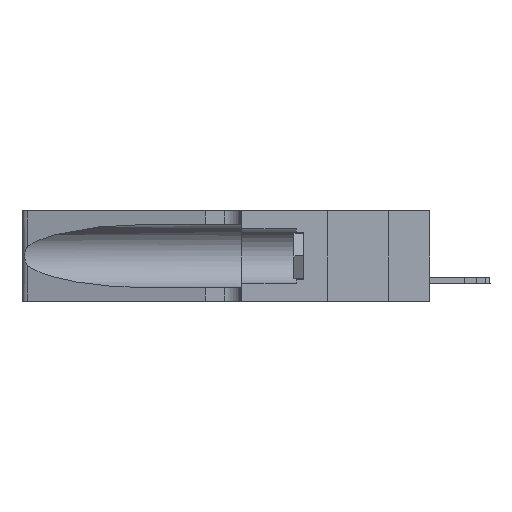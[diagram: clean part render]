
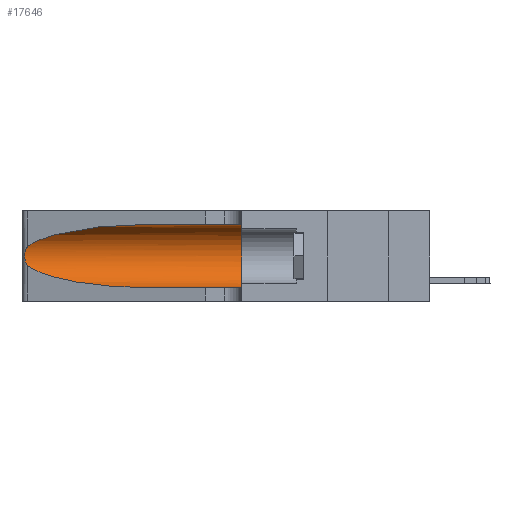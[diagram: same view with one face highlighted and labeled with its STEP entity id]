
A CAD part, left-side view. The second image highlights one B-rep face of the part: STEP entity #17646.
In plain terms, the highlighted cylindrical face has radius 3.308 mm (diameter 6.617 mm), a partial arc.
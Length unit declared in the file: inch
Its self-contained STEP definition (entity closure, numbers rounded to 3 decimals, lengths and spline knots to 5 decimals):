
#485 = ORIENTED_EDGE ( 'NONE', *, *, #11020, .T. ) ;
#548 =( BOUNDED_CURVE ( )  B_SPLINE_CURVE ( 3, ( #13055, #17147, #8443, #1246 ),
 .UNSPECIFIED., .F., .F. ) 
 B_SPLINE_CURVE_WITH_KNOTS ( ( 4, 4 ),
 ( 3.44316, 4.71239 ),
 .UNSPECIFIED. ) 
 CURVE ( )  GEOMETRIC_REPRESENTATION_ITEM ( )  RATIONAL_B_SPLINE_CURVE ( ( 1., 0.87, 0.87, 1. ) ) 
 REPRESENTATION_ITEM ( '' )  );
#1246 = CARTESIAN_POINT ( 'NONE',  ( 0.1305, 0.72297, 0.05475 ) ) ;
#1343 = CARTESIAN_POINT ( 'NONE',  ( 0.26075, 1.23896, 0.19203 ) ) ;
#1542 = CARTESIAN_POINT ( 'NONE',  ( 0.25856, 1.23593, 0.16098 ) ) ;
#1659 = CARTESIAN_POINT ( 'NONE',  ( 0.25487, 1.22718, 0.14631 ) ) ;
#2204 = DIRECTION ( 'NONE',  ( 0., 0., 1. ) ) ;
#2738 = CIRCLE ( 'NONE', #11949, 0.13025 ) ;
#2740 = CARTESIAN_POINT ( 'NONE',  ( 0.18966, 0.96281, 0.31525 ) ) ;
#3016 = VERTEX_POINT ( 'NONE', #12288 ) ;
#4189 = VERTEX_POINT ( 'NONE', #16537 ) ;
#4429 = CARTESIAN_POINT ( 'NONE',  ( 0.25789, 1.23486, 0.15765 ) ) ;
#4461 = EDGE_CURVE ( 'NONE', #3016, #16405, #2738, .T. ) ;
#4575 = CARTESIAN_POINT ( 'NONE',  ( 0.1305, 1.61858, 0.185 ) ) ;
#5717 = CARTESIAN_POINT ( 'NONE',  ( 0.25639, 1.23184, 0.21858 ) ) ;
#6683 = CARTESIAN_POINT ( 'NONE',  ( 0.1305, 0.35, 0.185 ) ) ;
#7173 = DIRECTION ( 'NONE',  ( 0., -1., 0. ) ) ;
#7194 = CARTESIAN_POINT ( 'NONE',  ( 0.25787, 1.23484, 0.2124 ) ) ;
#7376 = CARTESIAN_POINT ( 'NONE',  ( 0.26017, 1.23833, 0.17102 ) ) ;
#7525 = DIRECTION ( 'NONE',  ( 0., 0., -1. ) ) ;
#7537 = VECTOR ( 'NONE', #7173, 39.37008 ) ;
#7862 = LINE ( 'NONE', #10892, #14656 ) ;
#8037 = DIRECTION ( 'NONE',  ( 0., -1., 0. ) ) ;
#8443 = CARTESIAN_POINT ( 'NONE',  ( 0.18966, 0.96281, 0.05475 ) ) ;
#8663 = CARTESIAN_POINT ( 'NONE',  ( 0.25854, 1.2359, 0.20912 ) ) ;
#8679 = CYLINDRICAL_SURFACE ( 'NONE', #16673, 0.13025 ) ;
#9254 = CARTESIAN_POINT ( 'NONE',  ( 0.1305, 0.72297, 0.31525 ) ) ;
#9574 = CARTESIAN_POINT ( 'NONE',  ( 0.1305, 0.35, 0.05475 ) ) ;
#9608 = VERTEX_POINT ( 'NONE', #12617 ) ;
#9744 = EDGE_CURVE ( 'NONE', #11634, #9608, #17561, .T. ) ;
#10396 = ORIENTED_EDGE ( 'NONE', *, *, #11366, .F. ) ;
#10731 = LINE ( 'NONE', #13749, #7537 ) ;
#10815 = VERTEX_POINT ( 'NONE', #1659 ) ;
#10892 = CARTESIAN_POINT ( 'NONE',  ( 0.1305, 1.61858, 0.05475 ) ) ;
#11020 = EDGE_CURVE ( 'NONE', #10815, #4189, #548, .T. ) ;
#11366 = EDGE_CURVE ( 'NONE', #11634, #3016, #10731, .T. ) ;
#11390 = CARTESIAN_POINT ( 'NONE',  ( 0.25487, 1.22718, 0.22369 ) ) ;
#11634 = VERTEX_POINT ( 'NONE', #9254 ) ;
#11896 = EDGE_LOOP ( 'NONE', ( #17261, #17432, #485, #14064, #17115, #10396 ) ) ;
#11949 = AXIS2_PLACEMENT_3D ( 'NONE', #6683, #12455, #2204 ) ;
#12288 = CARTESIAN_POINT ( 'NONE',  ( 0.1305, 0.35, 0.31525 ) ) ;
#12455 = DIRECTION ( 'NONE',  ( 0., 1., 0. ) ) ;
#12617 = CARTESIAN_POINT ( 'NONE',  ( 0.25487, 1.22718, 0.22369 ) ) ;
#12893 = EDGE_CURVE ( 'NONE', #9608, #10815, #18157, .T. ) ;
#12911 = CARTESIAN_POINT ( 'NONE',  ( 0.2373, 1.15595, 0.28018 ) ) ;
#13055 = CARTESIAN_POINT ( 'NONE',  ( 0.25487, 1.22718, 0.14631 ) ) ;
#13416 = CARTESIAN_POINT ( 'NONE',  ( 0.25487, 1.22718, 0.22369 ) ) ;
#13749 = CARTESIAN_POINT ( 'NONE',  ( 0.1305, 1.61858, 0.31525 ) ) ;
#14064 = ORIENTED_EDGE ( 'NONE', *, *, #14989, .T. ) ;
#14421 = CARTESIAN_POINT ( 'NONE',  ( 0.25555, 1.22994, 0.2215 ) ) ;
#14552 = CARTESIAN_POINT ( 'NONE',  ( 0.26075, 1.23896, 0.178 ) ) ;
#14605 = CARTESIAN_POINT ( 'NONE',  ( 0.25639, 1.23186, 0.15144 ) ) ;
#14656 = VECTOR ( 'NONE', #8037, 39.37008 ) ;
#14730 = CARTESIAN_POINT ( 'NONE',  ( 0.25487, 1.22718, 0.14631 ) ) ;
#14989 = EDGE_CURVE ( 'NONE', #4189, #16405, #7862, .T. ) ;
#15617 = CARTESIAN_POINT ( 'NONE',  ( 0.1305, 0.72297, 0.31525 ) ) ;
#16259 = DIRECTION ( 'NONE',  ( 0., -1., 0. ) ) ;
#16405 = VERTEX_POINT ( 'NONE', #9574 ) ;
#16537 = CARTESIAN_POINT ( 'NONE',  ( 0.1305, 0.72297, 0.05475 ) ) ;
#16673 = AXIS2_PLACEMENT_3D ( 'NONE', #4575, #16259, #7525 ) ;
#17115 = ORIENTED_EDGE ( 'NONE', *, *, #4461, .F. ) ;
#17147 = CARTESIAN_POINT ( 'NONE',  ( 0.2373, 1.15595, 0.08982 ) ) ;
#17261 = ORIENTED_EDGE ( 'NONE', *, *, #9744, .T. ) ;
#17330 = FACE_OUTER_BOUND ( 'NONE', #11896, .T. ) ;
#17432 = ORIENTED_EDGE ( 'NONE', *, *, #12893, .T. ) ;
#17516 = CARTESIAN_POINT ( 'NONE',  ( 0.25555, 1.22993, 0.14849 ) ) ;
#17561 =( BOUNDED_CURVE ( )  B_SPLINE_CURVE ( 3, ( #15617, #2740, #12911, #13416 ),
 .UNSPECIFIED., .F., .T. ) 
 B_SPLINE_CURVE_WITH_KNOTS ( ( 4, 4 ),
 ( 1.5708, 2.84003 ),
 .UNSPECIFIED. ) 
 CURVE ( )  GEOMETRIC_REPRESENTATION_ITEM ( )  RATIONAL_B_SPLINE_CURVE ( ( 1., 0.87, 0.87, 1. ) ) 
 REPRESENTATION_ITEM ( '' )  );
#17646 = ADVANCED_FACE ( 'NONE', ( #17330 ), #8679, .F. ) ;
#18157 = B_SPLINE_CURVE_WITH_KNOTS ( 'NONE', 3,
 ( #11390, #14421, #5717, #7194, #8663, #18872, #1343, #14552, #7376, #1542, #4429, #14605, #17516, #14730 ),
 .UNSPECIFIED., .F., .F.,
 ( 4, 2, 2, 2, 2, 2, 4 ),
 ( 0., 0.00027, 0.00053, 0.00107, 0.0016, 0.00187, 0.00214 ),
 .UNSPECIFIED. ) ;
#18872 = CARTESIAN_POINT ( 'NONE',  ( 0.26018, 1.23835, 0.19895 ) ) ;
